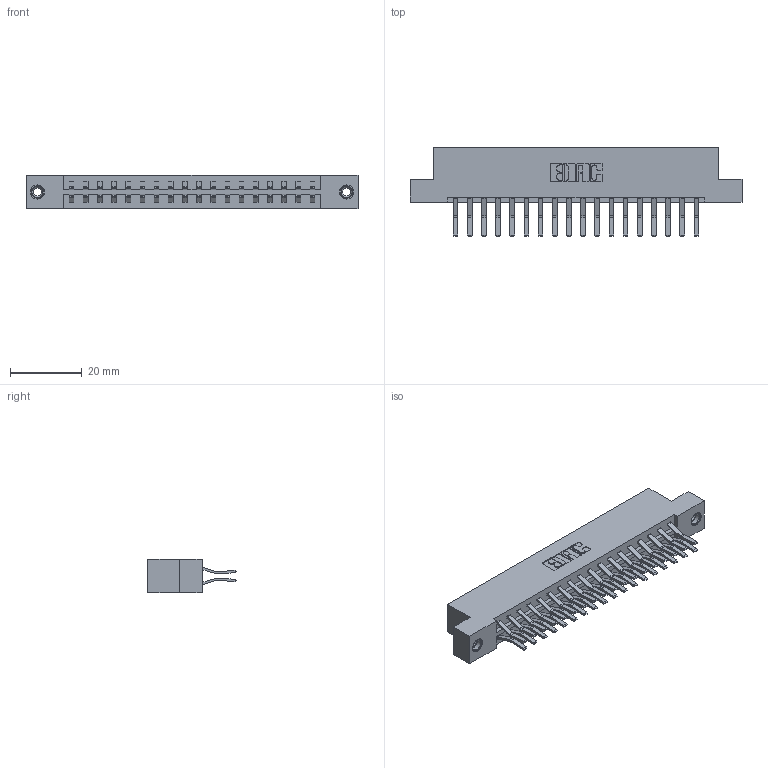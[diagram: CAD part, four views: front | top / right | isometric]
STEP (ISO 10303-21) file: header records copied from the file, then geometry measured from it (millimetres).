
FILE_DESCRIPTION (( 'STEP AP203' ), '1' );
FILE_NAME ('333-036-560-208.STEP', '2018-08-03T02:03:10', ( '' ), ( '' ), 'SwSTEP 2.0', 'SolidWorks 2016', '' );
FILE_SCHEMA (( 'CONFIG_CONTROL_DESIGN' ));
Length unit declared in the file: inch
Products named in the file (4): 345-292-001_560 Tail; 345-250-001_345-250-003-102; 333-036-560-208; 333 Part_Flush - .156 Dia - TI
Assembly tree (39 placements, depth 2):
  333-036-560-208
    333 Part_Flush - .156 Dia - TI
    345-292-001_560 Tail  x36
    345-250-001_345-250-003-102  x2
Bounding box: 92.86 x 24.78 x 9.4 mm (x, y, z)
Volume: 9485.7 mm3; surface area: 11651.5 mm2
Topology: 39 solids, 39 shells, 2118 faces, 6243 edges, 4106 vertices
Faces by surface type: plane 1398, cylinder 704, cone 12, torus 4
Entity records: 15958 total; most frequent: CARTESIAN_POINT 2657, ORIENTED_EDGE 2586, DIRECTION 2347, EDGE_CURVE 1293, VECTOR 1141, LINE 1141, VERTEX_POINT 856, AXIS2_PLACEMENT_3D 603
